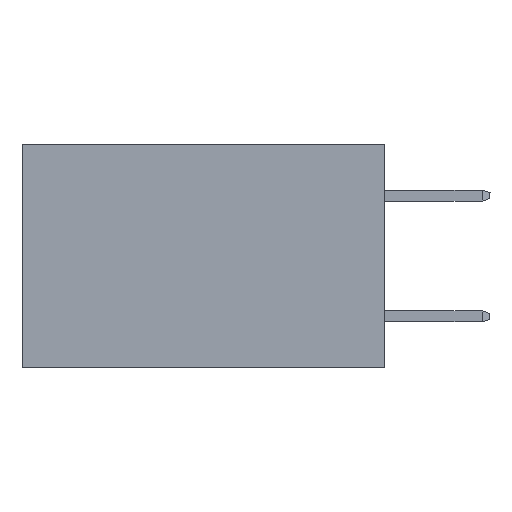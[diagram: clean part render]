
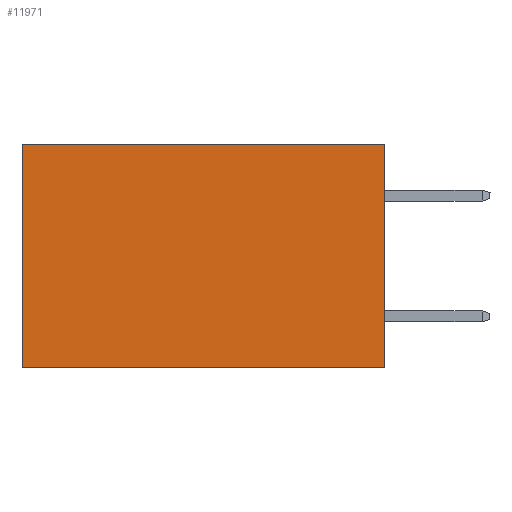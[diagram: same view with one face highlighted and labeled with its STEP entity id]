
A CAD part, left-side view. The second image highlights one B-rep face of the part: STEP entity #11971.
In plain terms, the highlighted planar face has unit normal (-1, 0, 0).
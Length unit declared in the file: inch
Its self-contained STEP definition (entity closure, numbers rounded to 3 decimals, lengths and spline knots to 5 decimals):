
#586 = ORIENTED_EDGE ( 'NONE', *, *, #12023, .F. ) ;
#665 = CARTESIAN_POINT ( 'NONE',  ( 0.298, 0., -0.37 ) ) ;
#786 = EDGE_CURVE ( 'NONE', #1568, #4518, #6869, .T. ) ;
#1243 = VERTEX_POINT ( 'NONE', #665 ) ;
#1385 = FACE_OUTER_BOUND ( 'NONE', #7029, .T. ) ;
#1568 = VERTEX_POINT ( 'NONE', #10518 ) ;
#2045 = CARTESIAN_POINT ( 'NONE',  ( 0.298, 0., 0. ) ) ;
#2064 = CARTESIAN_POINT ( 'NONE',  ( 0.298, 0., 0. ) ) ;
#2085 = DIRECTION ( 'NONE',  ( 0., 1., 0. ) ) ;
#2262 = LINE ( 'NONE', #6133, #7322 ) ;
#4518 = VERTEX_POINT ( 'NONE', #6011 ) ;
#4554 = VECTOR ( 'NONE', #10385, 39.37008 ) ;
#4648 = EDGE_CURVE ( 'NONE', #4518, #8482, #12395, .T. ) ;
#5736 = LINE ( 'NONE', #6012, #4554 ) ;
#6002 = CARTESIAN_POINT ( 'NONE',  ( 0.298, 0.6, -0.37 ) ) ;
#6011 = CARTESIAN_POINT ( 'NONE',  ( 0.298, 0.6, 0. ) ) ;
#6012 = CARTESIAN_POINT ( 'NONE',  ( 0.298, 0., 0. ) ) ;
#6133 = CARTESIAN_POINT ( 'NONE',  ( 0.298, 0., -0.37 ) ) ;
#6178 = PLANE ( 'NONE',  #12117 ) ;
#6869 = LINE ( 'NONE', #2064, #12480 ) ;
#7029 = EDGE_LOOP ( 'NONE', ( #7486, #7030, #586, #10154 ) ) ;
#7030 = ORIENTED_EDGE ( 'NONE', *, *, #9280, .F. ) ;
#7322 = VECTOR ( 'NONE', #2085, 39.37008 ) ;
#7418 = VECTOR ( 'NONE', #12359, 39.37008 ) ;
#7486 = ORIENTED_EDGE ( 'NONE', *, *, #4648, .T. ) ;
#8482 = VERTEX_POINT ( 'NONE', #6002 ) ;
#9280 = EDGE_CURVE ( 'NONE', #1243, #8482, #2262, .T. ) ;
#10069 = DIRECTION ( 'NONE',  ( 0., 1., 0. ) ) ;
#10092 = DIRECTION ( 'NONE',  ( 0., 0., -1. ) ) ;
#10154 = ORIENTED_EDGE ( 'NONE', *, *, #786, .T. ) ;
#10385 = DIRECTION ( 'NONE',  ( 0., 0., -1. ) ) ;
#10518 = CARTESIAN_POINT ( 'NONE',  ( 0.298, 0., 0. ) ) ;
#11343 = CARTESIAN_POINT ( 'NONE',  ( 0.298, 0.6, 0. ) ) ;
#11971 = ADVANCED_FACE ( 'NONE', ( #1385 ), #6178, .F. ) ;
#11988 = DIRECTION ( 'NONE',  ( 1., 0., 0. ) ) ;
#12023 = EDGE_CURVE ( 'NONE', #1568, #1243, #5736, .T. ) ;
#12117 = AXIS2_PLACEMENT_3D ( 'NONE', #2045, #11988, #10092 ) ;
#12359 = DIRECTION ( 'NONE',  ( 0., 0., -1. ) ) ;
#12395 = LINE ( 'NONE', #11343, #7418 ) ;
#12480 = VECTOR ( 'NONE', #10069, 39.37008 ) ;
